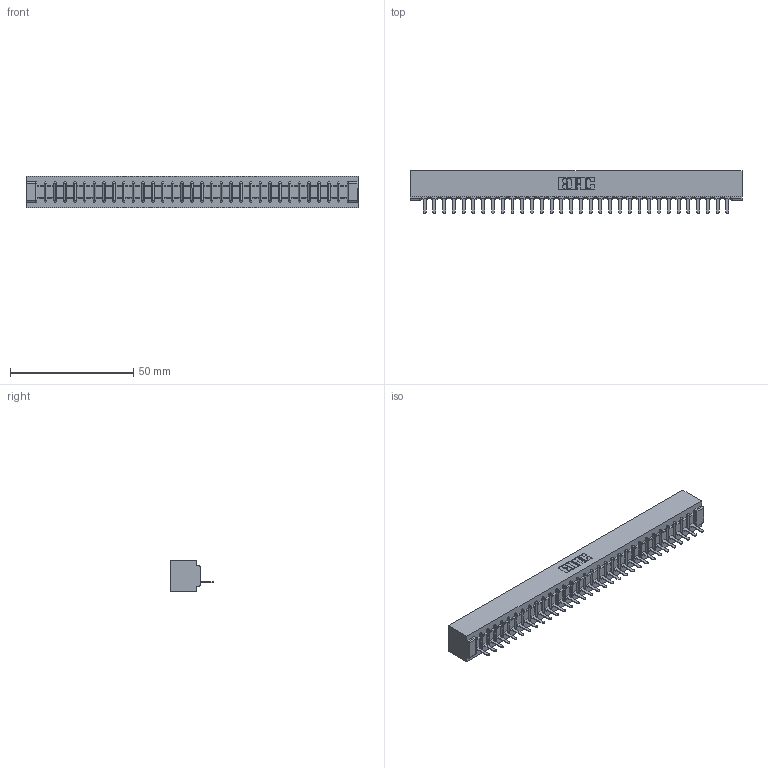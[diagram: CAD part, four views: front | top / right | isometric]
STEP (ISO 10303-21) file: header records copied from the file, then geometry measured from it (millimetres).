
FILE_DESCRIPTION (( 'STEP AP203' ), '1' );
FILE_NAME ('307-032-421-101.STEP', '2020-09-28T16:24:21', ( '' ), ( '' ), 'SwSTEP 2.0', 'SolidWorks 2020', '' );
FILE_SCHEMA (( 'CONFIG_CONTROL_DESIGN' ));
Length unit declared in the file: inch
Products named in the file (3): 307-032-421-101; 307 Part_No Mounting Lugs; 307-290-002_521
Assembly tree (33 placements, depth 2):
  307-032-421-101
    307 Part_No Mounting Lugs
    307-290-002_521  x32
Bounding box: 134.67 x 17.42 x 12.7 mm (x, y, z)
Volume: 14896.5 mm3; surface area: 18866.4 mm2
Topology: 33 solids, 33 shells, 2511 faces, 7723 edges, 5058 vertices
Faces by surface type: plane 1506, cylinder 939, sphere 66
Entity records: 29106 total; most frequent: CARTESIAN_POINT 4908, ORIENTED_EDGE 4898, DIRECTION 4771, EDGE_CURVE 2449, VECTOR 1873, LINE 1873, VERTEX_POINT 1586, AXIS2_PLACEMENT_3D 1449
